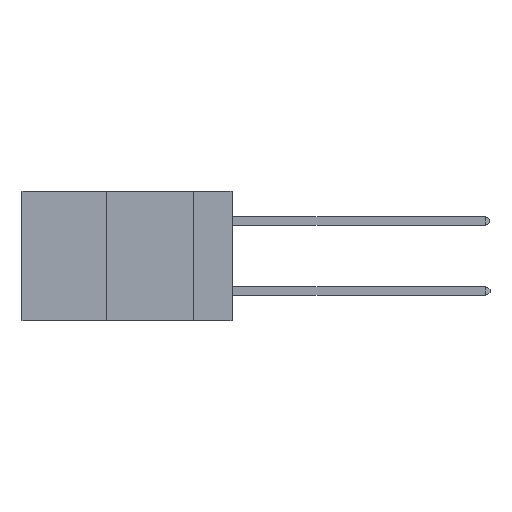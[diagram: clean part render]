
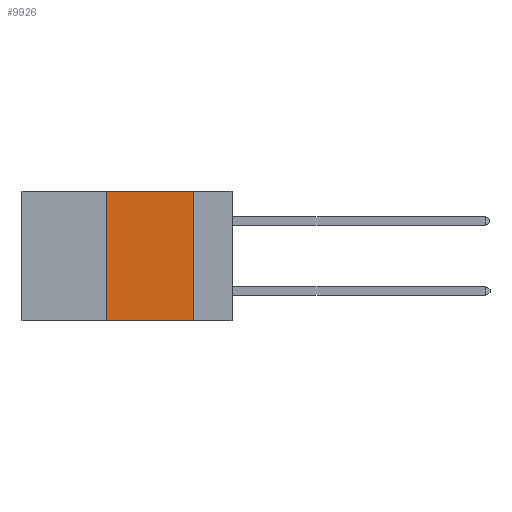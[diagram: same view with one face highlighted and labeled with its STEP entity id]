
A CAD part, left-side view. The second image highlights one B-rep face of the part: STEP entity #9926.
In plain terms, the highlighted planar face has unit normal (-1, 0, 0).
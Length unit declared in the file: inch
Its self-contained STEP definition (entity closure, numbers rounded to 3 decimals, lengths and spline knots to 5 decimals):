
#45 = ORIENTED_EDGE ( 'NONE', *, *, #11038, .F. ) ;
#661 = DIRECTION ( 'NONE',  ( 1., 0., 0. ) ) ;
#1071 = FACE_OUTER_BOUND ( 'NONE', #21580, .T. ) ;
#1146 = VECTOR ( 'NONE', #9017, 39.37008 ) ;
#1190 = VERTEX_POINT ( 'NONE', #18634 ) ;
#1440 = EDGE_CURVE ( 'NONE', #6176, #20482, #10998, .T. ) ;
#1449 = DIRECTION ( 'NONE',  ( 0., 0., -1. ) ) ;
#1690 = LINE ( 'NONE', #17411, #1146 ) ;
#1753 = ORIENTED_EDGE ( 'NONE', *, *, #15146, .T. ) ;
#2035 = AXIS2_PLACEMENT_3D ( 'NONE', #10850, #661, #12550 ) ;
#2329 = EDGE_CURVE ( 'NONE', #1190, #19524, #12546, .T. ) ;
#6176 = VERTEX_POINT ( 'NONE', #7204 ) ;
#7204 = CARTESIAN_POINT ( 'NONE',  ( 0., 0.11, 0. ) ) ;
#7767 = VECTOR ( 'NONE', #9609, 39.37008 ) ;
#9017 = DIRECTION ( 'NONE',  ( 0., -1., 0. ) ) ;
#9609 = DIRECTION ( 'NONE',  ( 0., -1., 0. ) ) ;
#9926 = ADVANCED_FACE ( 'NONE', ( #1071 ), #20918, .F. ) ;
#10850 = CARTESIAN_POINT ( 'NONE',  ( 0., 0.6, 0. ) ) ;
#10998 = LINE ( 'NONE', #16405, #15474 ) ;
#11038 = EDGE_CURVE ( 'NONE', #19524, #6176, #12136, .T. ) ;
#12136 = LINE ( 'NONE', #17978, #7767 ) ;
#12546 = LINE ( 'NONE', #21460, #16516 ) ;
#12550 = DIRECTION ( 'NONE',  ( 0., 0., -1. ) ) ;
#15131 = CARTESIAN_POINT ( 'NONE',  ( 0., 0.36, 0. ) ) ;
#15146 = EDGE_CURVE ( 'NONE', #1190, #20482, #1690, .T. ) ;
#15474 = VECTOR ( 'NONE', #1449, 39.37008 ) ;
#16035 = ORIENTED_EDGE ( 'NONE', *, *, #1440, .F. ) ;
#16405 = CARTESIAN_POINT ( 'NONE',  ( 0., 0.11, 0. ) ) ;
#16516 = VECTOR ( 'NONE', #18125, 39.37008 ) ;
#17411 = CARTESIAN_POINT ( 'NONE',  ( 0., 0.6, -0.37 ) ) ;
#17978 = CARTESIAN_POINT ( 'NONE',  ( 0., 0.6, 0. ) ) ;
#18125 = DIRECTION ( 'NONE',  ( 0., 0., 1. ) ) ;
#18613 = ORIENTED_EDGE ( 'NONE', *, *, #2329, .F. ) ;
#18634 = CARTESIAN_POINT ( 'NONE',  ( 0., 0.36, -0.37 ) ) ;
#19357 = CARTESIAN_POINT ( 'NONE',  ( 0., 0.11, -0.37 ) ) ;
#19524 = VERTEX_POINT ( 'NONE', #15131 ) ;
#20482 = VERTEX_POINT ( 'NONE', #19357 ) ;
#20918 = PLANE ( 'NONE',  #2035 ) ;
#21460 = CARTESIAN_POINT ( 'NONE',  ( 0., 0.36, 0. ) ) ;
#21580 = EDGE_LOOP ( 'NONE', ( #16035, #45, #18613, #1753 ) ) ;
